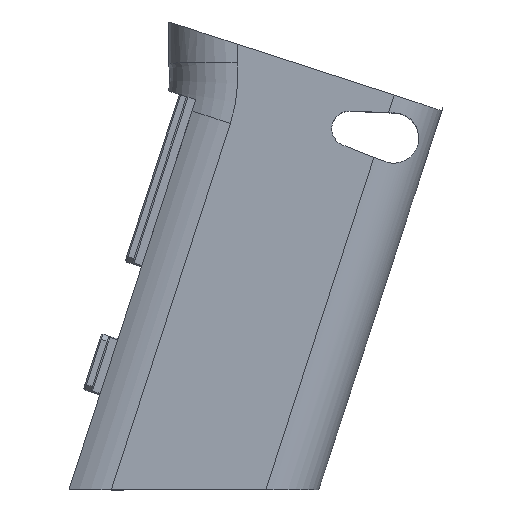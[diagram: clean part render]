
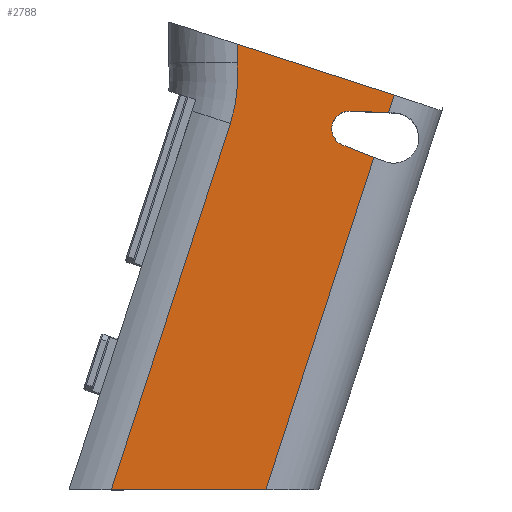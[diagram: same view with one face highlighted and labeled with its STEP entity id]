
A CAD part, top view. The second image highlights one B-rep face of the part: STEP entity #2788.
In plain terms, the highlighted planar face has unit normal (0, 0, 1).
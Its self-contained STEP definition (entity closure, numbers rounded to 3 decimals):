
#134=FACE_OUTER_BOUND('',#285,.T.);
#285=EDGE_LOOP('',(#1885,#1886,#1887,#1888,#1889,#1890,#1891,#1892,#1893,
#1894));
#434=CIRCLE('',#3001,27.537);
#435=CIRCLE('',#3002,3.25);
#474=LINE('',#4033,#802);
#499=LINE('',#4111,#827);
#500=LINE('',#4144,#828);
#504=LINE('',#4182,#832);
#505=LINE('',#4186,#833);
#506=LINE('',#4187,#834);
#507=LINE('',#4189,#835);
#508=LINE('',#4192,#836);
#802=VECTOR('',#3229,10.);
#827=VECTOR('',#3282,10.);
#828=VECTOR('',#3287,10.);
#832=VECTOR('',#3297,10.);
#833=VECTOR('',#3300,10.);
#834=VECTOR('',#3301,10.);
#835=VECTOR('',#3302,10.);
#836=VECTOR('',#3305,10.);
#1130=VERTEX_POINT('',#4018);
#1132=VERTEX_POINT('',#4032);
#1159=VERTEX_POINT('',#4110);
#1162=VERTEX_POINT('',#4141);
#1163=VERTEX_POINT('',#4143);
#1170=VERTEX_POINT('',#4181);
#1171=VERTEX_POINT('',#4183);
#1172=VERTEX_POINT('',#4185);
#1173=VERTEX_POINT('',#4188);
#1174=VERTEX_POINT('',#4190);
#1404=EDGE_CURVE('',#1132,#1130,#474,.T.);
#1438=EDGE_CURVE('',#1132,#1159,#499,.T.);
#1442=EDGE_CURVE('',#1162,#1163,#500,.T.);
#1450=EDGE_CURVE('',#1170,#1130,#504,.T.);
#1451=EDGE_CURVE('',#1171,#1170,#434,.T.);
#1452=EDGE_CURVE('',#1172,#1171,#505,.T.);
#1453=EDGE_CURVE('',#1163,#1172,#506,.T.);
#1454=EDGE_CURVE('',#1162,#1173,#507,.T.);
#1455=EDGE_CURVE('',#1173,#1174,#435,.T.);
#1456=EDGE_CURVE('',#1174,#1159,#508,.T.);
#1885=ORIENTED_EDGE('',*,*,#1404,.T.);
#1886=ORIENTED_EDGE('',*,*,#1450,.F.);
#1887=ORIENTED_EDGE('',*,*,#1451,.F.);
#1888=ORIENTED_EDGE('',*,*,#1452,.F.);
#1889=ORIENTED_EDGE('',*,*,#1453,.F.);
#1890=ORIENTED_EDGE('',*,*,#1442,.F.);
#1891=ORIENTED_EDGE('',*,*,#1454,.T.);
#1892=ORIENTED_EDGE('',*,*,#1455,.T.);
#1893=ORIENTED_EDGE('',*,*,#1456,.T.);
#1894=ORIENTED_EDGE('',*,*,#1438,.F.);
#2665=PLANE('',#3000);
#2788=ADVANCED_FACE('',(#134),#2665,.F.);
#3000=AXIS2_PLACEMENT_3D('',#4180,#3295,#3296);
#3001=AXIS2_PLACEMENT_3D('',#4184,#3298,#3299);
#3002=AXIS2_PLACEMENT_3D('',#4191,#3303,#3304);
#3229=DIRECTION('',(-0.951,0.309,0.));
#3282=DIRECTION('',(-0.309,-0.951,0.));
#3287=DIRECTION('',(-0.309,-0.951,0.));
#3295=DIRECTION('center_axis',(0.,0.,
-1.));
#3296=DIRECTION('ref_axis',(1.,0.,0.));
#3297=DIRECTION('',(0.,1.,0.));
#3298=DIRECTION('center_axis',(0.,0.,
1.));
#3299=DIRECTION('ref_axis',(0.93,0.368,0.));
#3300=DIRECTION('',(0.309,0.951,0.));
#3301=DIRECTION('',(-1.,0.,0.));
#3302=DIRECTION('',(-0.931,0.364,0.));
#3303=DIRECTION('center_axis',(0.,0.,
-1.));
#3304=DIRECTION('ref_axis',(1.,0.,0.));
#3305=DIRECTION('',(0.999,-0.041,0.));
#4018=CARTESIAN_POINT('',(-51.645,31.84,-5.));
#4032=CARTESIAN_POINT('',(-22.717,22.441,-5.));
#4033=CARTESIAN_POINT('',(-70.647,38.014,-5.));
#4110=CARTESIAN_POINT('',(-23.766,19.213,-5.));
#4111=CARTESIAN_POINT('',(-21.646,25.738,-5.));
#4141=CARTESIAN_POINT('',(-26.435,11.,-5.));
#4143=CARTESIAN_POINT('',(-46.329,-50.229,-5.));
#4144=CARTESIAN_POINT('',(-21.646,25.738,-5.));
#4180=CARTESIAN_POINT('Origin',(-97.655,53.375,-5.));
#4181=CARTESIAN_POINT('',(-51.645,28.375,-5.));
#4182=CARTESIAN_POINT('',(-51.645,28.375,-5.));
#4183=CARTESIAN_POINT('',(-52.867,17.237,-5.));
#4184=CARTESIAN_POINT('Origin',(-79.057,25.747,-5.));
#4185=CARTESIAN_POINT('',(-74.788,-50.229,-5.));
#4186=CARTESIAN_POINT('',(-61.283,-8.665,-5.));
#4187=CARTESIAN_POINT('',(-66.453,-50.229,-5.));
#4188=CARTESIAN_POINT('',(-32.137,13.229,-5.));
#4189=CARTESIAN_POINT('',(-63.533,25.5,-5.));
#4190=CARTESIAN_POINT('',(-30.821,19.503,-5.));
#4191=CARTESIAN_POINT('Origin',(-30.954,16.256,-5.));
#4192=CARTESIAN_POINT('',(-64.876,20.903,-5.));
